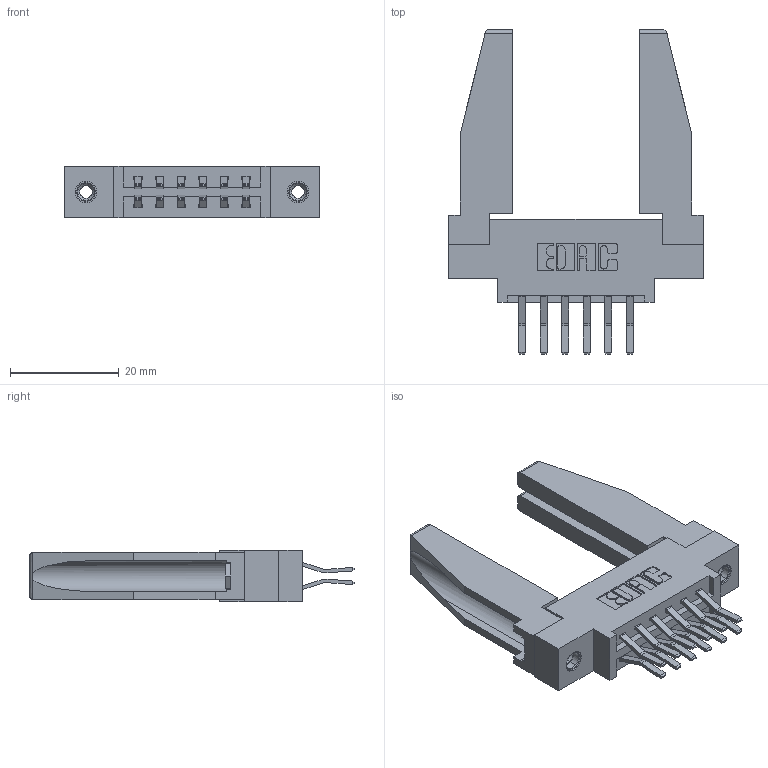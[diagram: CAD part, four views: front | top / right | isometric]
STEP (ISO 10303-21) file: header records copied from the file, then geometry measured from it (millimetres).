
FILE_DESCRIPTION (( 'STEP AP203' ), '1' );
FILE_NAME ('337-012-560-878.STEP', '2019-10-10T16:33:39', ( '' ), ( '' ), 'SwSTEP 2.0', 'SolidWorks 2016', '' );
FILE_SCHEMA (( 'CONFIG_CONTROL_DESIGN' ));
Length unit declared in the file: inch
Products named in the file (5): 337 Part_0.170 Offset - 0.156 Dia-TI; 337-012-560-878; 345-250-001_345-250-001-102; 345-292-001_560 Tail; 307-220-078
Assembly tree (17 placements, depth 2):
  337-012-560-878
    337 Part_0.170 Offset - 0.156 Dia-TI
    345-292-001_560 Tail  x12
    345-250-001_345-250-001-102  x2
    307-220-078  x2
Bounding box: 46.79 x 59.58 x 9.4 mm (x, y, z)
Volume: 8406 mm3; surface area: 8804.8 mm2
Topology: 17 solids, 17 shells, 920 faces, 2657 edges, 1746 vertices
Faces by surface type: plane 614, cylinder 290, cone 12, torus 4
Entity records: 11968 total; most frequent: CARTESIAN_POINT 2048, ORIENTED_EDGE 1940, DIRECTION 1818, EDGE_CURVE 970, VECTOR 800, LINE 800, VERTEX_POINT 640, AXIS2_PLACEMENT_3D 509
